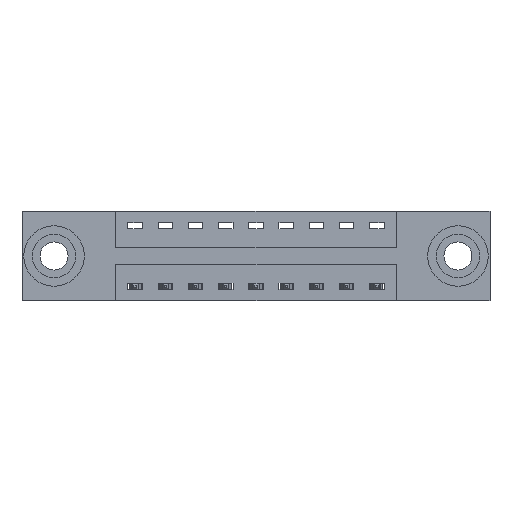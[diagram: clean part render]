
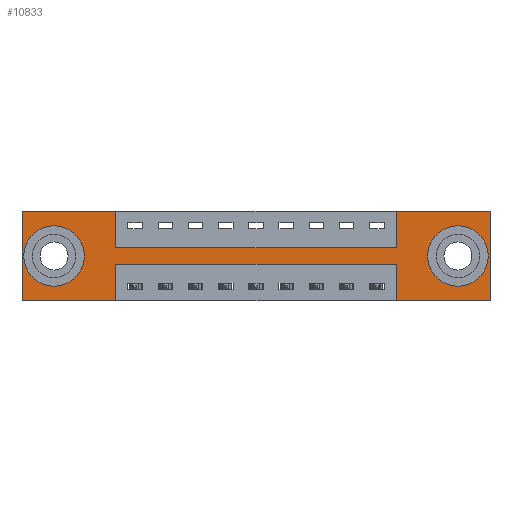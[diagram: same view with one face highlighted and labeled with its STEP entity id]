
A CAD part, front view. The second image highlights one B-rep face of the part: STEP entity #10833.
In plain terms, the highlighted planar face has unit normal (0, -1, 0).
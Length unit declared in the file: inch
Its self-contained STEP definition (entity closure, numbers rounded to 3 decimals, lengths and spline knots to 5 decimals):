
#7 = DIRECTION ( 'NONE',  ( 0., 1., 0. ) ) ;
#70 = ORIENTED_EDGE ( 'NONE', *, *, #6863, .F. ) ;
#81 = LINE ( 'NONE', #3371, #8664 ) ;
#238 = VERTEX_POINT ( 'NONE', #8676 ) ;
#256 = CARTESIAN_POINT ( 'NONE',  ( 1.5475, 0., 0. ) ) ;
#318 = VECTOR ( 'NONE', #4510, 39.37008 ) ;
#411 = EDGE_CURVE ( 'NONE', #2288, #8568, #5876, .T. ) ;
#420 = ORIENTED_EDGE ( 'NONE', *, *, #6137, .F. ) ;
#549 = EDGE_CURVE ( 'NONE', #10380, #238, #9472, .T. ) ;
#562 = CARTESIAN_POINT ( 'NONE',  ( 0., 0., 0. ) ) ;
#576 = DIRECTION ( 'NONE',  ( 0., 0., 1. ) ) ;
#618 = CARTESIAN_POINT ( 'NONE',  ( 0., 0., -0.37 ) ) ;
#656 = CARTESIAN_POINT ( 'NONE',  ( 0.3875, 0., -0.22 ) ) ;
#703 = DIRECTION ( 'NONE',  ( 0., 1., 0. ) ) ;
#706 = CARTESIAN_POINT ( 'NONE',  ( 0.3875, 0., -0.22 ) ) ;
#1052 = AXIS2_PLACEMENT_3D ( 'NONE', #2354, #703, #1323 ) ;
#1209 = VECTOR ( 'NONE', #4353, 39.37008 ) ;
#1259 = CARTESIAN_POINT ( 'NONE',  ( 0., 0., 0. ) ) ;
#1323 = DIRECTION ( 'NONE',  ( 0., 0., -1. ) ) ;
#1383 = LINE ( 'NONE', #8116, #2400 ) ;
#1456 = DIRECTION ( 'NONE',  ( 0., 0., 1. ) ) ;
#1584 = CARTESIAN_POINT ( 'NONE',  ( 1.935, 0., 0. ) ) ;
#1591 = EDGE_CURVE ( 'NONE', #2062, #9630, #2592, .T. ) ;
#1598 = VECTOR ( 'NONE', #8559, 39.37008 ) ;
#1780 = VERTEX_POINT ( 'NONE', #4697 ) ;
#1953 = ORIENTED_EDGE ( 'NONE', *, *, #5249, .F. ) ;
#1980 = ORIENTED_EDGE ( 'NONE', *, *, #10550, .F. ) ;
#2062 = VERTEX_POINT ( 'NONE', #7500 ) ;
#2075 = EDGE_CURVE ( 'NONE', #2584, #2062, #2580, .T. ) ;
#2124 = VERTEX_POINT ( 'NONE', #5237 ) ;
#2288 = VERTEX_POINT ( 'NONE', #8386 ) ;
#2354 = CARTESIAN_POINT ( 'NONE',  ( 1.8025, 0., -0.185 ) ) ;
#2381 = VECTOR ( 'NONE', #5872, 39.37008 ) ;
#2400 = VECTOR ( 'NONE', #10043, 39.37008 ) ;
#2410 = AXIS2_PLACEMENT_3D ( 'NONE', #6629, #4018, #5831 ) ;
#2580 = LINE ( 'NONE', #10313, #318 ) ;
#2584 = VERTEX_POINT ( 'NONE', #5385 ) ;
#2592 = LINE ( 'NONE', #256, #1209 ) ;
#2644 = DIRECTION ( 'NONE',  ( 0., 0., 1. ) ) ;
#2704 = CIRCLE ( 'NONE', #3781, 0.078 ) ;
#2710 = VECTOR ( 'NONE', #1456, 39.37008 ) ;
#3106 = DIRECTION ( 'NONE',  ( -1., 0., 0. ) ) ;
#3371 = CARTESIAN_POINT ( 'NONE',  ( 1.5475, 0., -0.37 ) ) ;
#3614 = EDGE_LOOP ( 'NONE', ( #1980, #8431, #70, #420, #8671, #6961, #6446, #5609, #7648, #10036, #9199, #1953 ) ) ;
#3706 = VERTEX_POINT ( 'NONE', #706 ) ;
#3781 = AXIS2_PLACEMENT_3D ( 'NONE', #10077, #10917, #576 ) ;
#4018 = DIRECTION ( 'NONE',  ( 0., -1., 0. ) ) ;
#4076 = FACE_BOUND ( 'NONE', #7890, .T. ) ;
#4208 = CARTESIAN_POINT ( 'NONE',  ( 0.1325, 0., -0.263 ) ) ;
#4353 = DIRECTION ( 'NONE',  ( 0., 0., 1. ) ) ;
#4374 = AXIS2_PLACEMENT_3D ( 'NONE', #8687, #10261, #2644 ) ;
#4510 = DIRECTION ( 'NONE',  ( 1., 0., 0. ) ) ;
#4697 = CARTESIAN_POINT ( 'NONE',  ( 1.935, 0., -0.37 ) ) ;
#4803 = VERTEX_POINT ( 'NONE', #9162 ) ;
#4864 = CIRCLE ( 'NONE', #8641, 0.078 ) ;
#4876 = VECTOR ( 'NONE', #10044, 39.37008 ) ;
#4938 = FACE_BOUND ( 'NONE', #10013, .T. ) ;
#4957 = CARTESIAN_POINT ( 'NONE',  ( 0., 0., -0.37 ) ) ;
#4982 = EDGE_CURVE ( 'NONE', #8568, #2288, #4864, .T. ) ;
#5110 = ORIENTED_EDGE ( 'NONE', *, *, #4982, .T. ) ;
#5237 = CARTESIAN_POINT ( 'NONE',  ( 0., 0., -0.37 ) ) ;
#5249 = EDGE_CURVE ( 'NONE', #5489, #2124, #5693, .T. ) ;
#5317 = DIRECTION ( 'NONE',  ( 0., 0., -1. ) ) ;
#5347 = EDGE_CURVE ( 'NONE', #8575, #1780, #9203, .T. ) ;
#5385 = CARTESIAN_POINT ( 'NONE',  ( 0.3875, 0., -0.15 ) ) ;
#5448 = VERTEX_POINT ( 'NONE', #4208 ) ;
#5469 = VECTOR ( 'NONE', #5317, 39.37008 ) ;
#5489 = VERTEX_POINT ( 'NONE', #7639 ) ;
#5552 = CARTESIAN_POINT ( 'NONE',  ( 0.3875, 0., 0. ) ) ;
#5609 = ORIENTED_EDGE ( 'NONE', *, *, #2075, .F. ) ;
#5660 = CARTESIAN_POINT ( 'NONE',  ( 1.8025, 0., -0.107 ) ) ;
#5693 = LINE ( 'NONE', #4957, #7027 ) ;
#5726 = EDGE_CURVE ( 'NONE', #5448, #8366, #2704, .T. ) ;
#5783 = VECTOR ( 'NONE', #9176, 39.37008 ) ;
#5831 = DIRECTION ( 'NONE',  ( 0., 0., -1. ) ) ;
#5872 = DIRECTION ( 'NONE',  ( 1., 0., 0. ) ) ;
#5876 = CIRCLE ( 'NONE', #1052, 0.078 ) ;
#6047 = EDGE_CURVE ( 'NONE', #2124, #10380, #10790, .T. ) ;
#6137 = EDGE_CURVE ( 'NONE', #1780, #9530, #6623, .T. ) ;
#6200 = DIRECTION ( 'NONE',  ( 0., 0., -1. ) ) ;
#6446 = ORIENTED_EDGE ( 'NONE', *, *, #1591, .F. ) ;
#6456 = CARTESIAN_POINT ( 'NONE',  ( 0., 0., 0. ) ) ;
#6623 = LINE ( 'NONE', #618, #5783 ) ;
#6629 = CARTESIAN_POINT ( 'NONE',  ( 0., 0., -0.37 ) ) ;
#6863 = EDGE_CURVE ( 'NONE', #9530, #4803, #81, .T. ) ;
#6873 = ORIENTED_EDGE ( 'NONE', *, *, #9935, .T. ) ;
#6887 = DIRECTION ( 'NONE',  ( 0., 0., 1. ) ) ;
#6961 = ORIENTED_EDGE ( 'NONE', *, *, #9762, .F. ) ;
#7027 = VECTOR ( 'NONE', #9097, 39.37008 ) ;
#7462 = LINE ( 'NONE', #562, #2381 ) ;
#7500 = CARTESIAN_POINT ( 'NONE',  ( 1.5475, 0., -0.15 ) ) ;
#7616 = CARTESIAN_POINT ( 'NONE',  ( 0.1325, 0., -0.107 ) ) ;
#7639 = CARTESIAN_POINT ( 'NONE',  ( 0.3875, 0., -0.37 ) ) ;
#7648 = ORIENTED_EDGE ( 'NONE', *, *, #8475, .F. ) ;
#7890 = EDGE_LOOP ( 'NONE', ( #6873, #8470 ) ) ;
#8027 = LINE ( 'NONE', #5552, #5469 ) ;
#8116 = CARTESIAN_POINT ( 'NONE',  ( 0.3875, 0., -0.37 ) ) ;
#8366 = VERTEX_POINT ( 'NONE', #7616 ) ;
#8386 = CARTESIAN_POINT ( 'NONE',  ( 1.8025, 0., -0.263 ) ) ;
#8431 = ORIENTED_EDGE ( 'NONE', *, *, #10189, .F. ) ;
#8470 = ORIENTED_EDGE ( 'NONE', *, *, #5726, .T. ) ;
#8475 = EDGE_CURVE ( 'NONE', #238, #2584, #8027, .T. ) ;
#8559 = DIRECTION ( 'NONE',  ( 1., 0., 0. ) ) ;
#8568 = VERTEX_POINT ( 'NONE', #5660 ) ;
#8575 = VERTEX_POINT ( 'NONE', #10109 ) ;
#8641 = AXIS2_PLACEMENT_3D ( 'NONE', #8736, #7, #6200 ) ;
#8664 = VECTOR ( 'NONE', #6887, 39.37008 ) ;
#8671 = ORIENTED_EDGE ( 'NONE', *, *, #5347, .F. ) ;
#8676 = CARTESIAN_POINT ( 'NONE',  ( 0.3875, 0., 0. ) ) ;
#8687 = CARTESIAN_POINT ( 'NONE',  ( 0.1325, 0., -0.185 ) ) ;
#8698 = VECTOR ( 'NONE', #3106, 39.37008 ) ;
#8736 = CARTESIAN_POINT ( 'NONE',  ( 1.8025, 0., -0.185 ) ) ;
#8738 = ORIENTED_EDGE ( 'NONE', *, *, #411, .T. ) ;
#9097 = DIRECTION ( 'NONE',  ( -1., 0., 0. ) ) ;
#9129 = PLANE ( 'NONE',  #2410 ) ;
#9162 = CARTESIAN_POINT ( 'NONE',  ( 1.5475, 0., -0.22 ) ) ;
#9176 = DIRECTION ( 'NONE',  ( -1., 0., 0. ) ) ;
#9199 = ORIENTED_EDGE ( 'NONE', *, *, #6047, .F. ) ;
#9203 = LINE ( 'NONE', #1584, #4876 ) ;
#9472 = LINE ( 'NONE', #10241, #1598 ) ;
#9530 = VERTEX_POINT ( 'NONE', #9636 ) ;
#9630 = VERTEX_POINT ( 'NONE', #9851 ) ;
#9636 = CARTESIAN_POINT ( 'NONE',  ( 1.5475, 0., -0.37 ) ) ;
#9762 = EDGE_CURVE ( 'NONE', #9630, #8575, #7462, .T. ) ;
#9851 = CARTESIAN_POINT ( 'NONE',  ( 1.5475, 0., 0. ) ) ;
#9935 = EDGE_CURVE ( 'NONE', #8366, #5448, #10508, .T. ) ;
#10013 = EDGE_LOOP ( 'NONE', ( #5110, #8738 ) ) ;
#10024 = FACE_OUTER_BOUND ( 'NONE', #3614, .T. ) ;
#10036 = ORIENTED_EDGE ( 'NONE', *, *, #549, .F. ) ;
#10043 = DIRECTION ( 'NONE',  ( 0., 0., -1. ) ) ;
#10044 = DIRECTION ( 'NONE',  ( 0., 0., -1. ) ) ;
#10077 = CARTESIAN_POINT ( 'NONE',  ( 0.1325, 0., -0.185 ) ) ;
#10109 = CARTESIAN_POINT ( 'NONE',  ( 1.935, 0., 0. ) ) ;
#10189 = EDGE_CURVE ( 'NONE', #4803, #3706, #10829, .T. ) ;
#10241 = CARTESIAN_POINT ( 'NONE',  ( 0., 0., 0. ) ) ;
#10261 = DIRECTION ( 'NONE',  ( 0., 1., 0. ) ) ;
#10313 = CARTESIAN_POINT ( 'NONE',  ( 0.3875, 0., -0.15 ) ) ;
#10380 = VERTEX_POINT ( 'NONE', #1259 ) ;
#10508 = CIRCLE ( 'NONE', #4374, 0.078 ) ;
#10550 = EDGE_CURVE ( 'NONE', #3706, #5489, #1383, .T. ) ;
#10790 = LINE ( 'NONE', #6456, #2710 ) ;
#10829 = LINE ( 'NONE', #656, #8698 ) ;
#10833 = ADVANCED_FACE ( 'NONE', ( #4938, #4076, #10024 ), #9129, .T. ) ;
#10917 = DIRECTION ( 'NONE',  ( 0., 1., 0. ) ) ;
